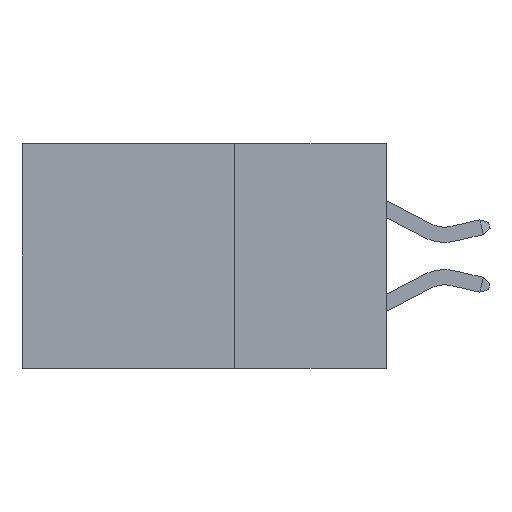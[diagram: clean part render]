
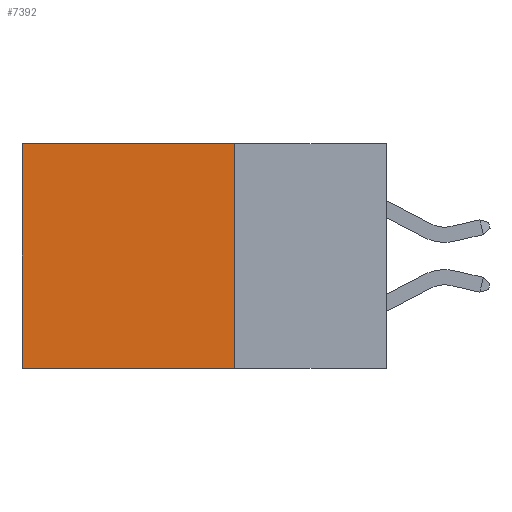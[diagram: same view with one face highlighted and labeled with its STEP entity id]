
A CAD part, left-side view. The second image highlights one B-rep face of the part: STEP entity #7392.
In plain terms, the highlighted planar face has unit normal (-1, 0, 0).
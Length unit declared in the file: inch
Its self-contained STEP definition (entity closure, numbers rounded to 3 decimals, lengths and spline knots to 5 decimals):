
#313 = EDGE_LOOP ( 'NONE', ( #14662, #8464, #5794, #7870 ) ) ;
#520 = CARTESIAN_POINT ( 'NONE',  ( 0.298, 0.25, 0. ) ) ;
#946 = DIRECTION ( 'NONE',  ( 0., 1., 0. ) ) ;
#1087 = DIRECTION ( 'NONE',  ( 0., 0., -1. ) ) ;
#1843 = DIRECTION ( 'NONE',  ( 0., 0., -1. ) ) ;
#2700 = VECTOR ( 'NONE', #10685, 39.37008 ) ;
#3041 = CARTESIAN_POINT ( 'NONE',  ( 0.298, 0.25, 0. ) ) ;
#3548 = CARTESIAN_POINT ( 'NONE',  ( 0.298, 0.25, -0.37 ) ) ;
#4116 = VERTEX_POINT ( 'NONE', #3548 ) ;
#4479 = CARTESIAN_POINT ( 'NONE',  ( 0.298, 0.25, 0. ) ) ;
#5794 = ORIENTED_EDGE ( 'NONE', *, *, #16434, .F. ) ;
#6106 = LINE ( 'NONE', #3041, #2700 ) ;
#7392 = ADVANCED_FACE ( 'NONE', ( #7986 ), #8253, .F. ) ;
#7409 = CARTESIAN_POINT ( 'NONE',  ( 0.298, 0.25, -0.37 ) ) ;
#7536 = CARTESIAN_POINT ( 'NONE',  ( 0.298, 0.6, 0. ) ) ;
#7870 = ORIENTED_EDGE ( 'NONE', *, *, #9938, .T. ) ;
#7986 = FACE_OUTER_BOUND ( 'NONE', #313, .T. ) ;
#8253 = PLANE ( 'NONE',  #8782 ) ;
#8284 = VECTOR ( 'NONE', #10063, 39.37008 ) ;
#8464 = ORIENTED_EDGE ( 'NONE', *, *, #12519, .F. ) ;
#8722 = CARTESIAN_POINT ( 'NONE',  ( 0.298, 0.6, -0.37 ) ) ;
#8782 = AXIS2_PLACEMENT_3D ( 'NONE', #520, #9537, #1843 ) ;
#8989 = VERTEX_POINT ( 'NONE', #11101 ) ;
#9472 = VERTEX_POINT ( 'NONE', #4479 ) ;
#9537 = DIRECTION ( 'NONE',  ( 1., 0., 0. ) ) ;
#9938 = EDGE_CURVE ( 'NONE', #9472, #8989, #6106, .T. ) ;
#10063 = DIRECTION ( 'NONE',  ( 0., 0., -1. ) ) ;
#10158 = VECTOR ( 'NONE', #1087, 39.37008 ) ;
#10562 = LINE ( 'NONE', #7536, #10158 ) ;
#10685 = DIRECTION ( 'NONE',  ( 0., 1., 0. ) ) ;
#11101 = CARTESIAN_POINT ( 'NONE',  ( 0.298, 0.6, 0. ) ) ;
#12519 = EDGE_CURVE ( 'NONE', #4116, #16401, #13626, .T. ) ;
#13626 = LINE ( 'NONE', #7409, #14055 ) ;
#13811 = EDGE_CURVE ( 'NONE', #8989, #16401, #10562, .T. ) ;
#14055 = VECTOR ( 'NONE', #946, 39.37008 ) ;
#14662 = ORIENTED_EDGE ( 'NONE', *, *, #13811, .T. ) ;
#15126 = LINE ( 'NONE', #15199, #8284 ) ;
#15199 = CARTESIAN_POINT ( 'NONE',  ( 0.298, 0.25, 0. ) ) ;
#16401 = VERTEX_POINT ( 'NONE', #8722 ) ;
#16434 = EDGE_CURVE ( 'NONE', #9472, #4116, #15126, .T. ) ;
